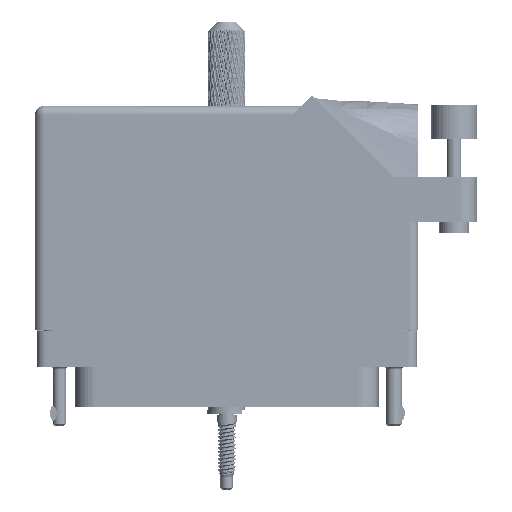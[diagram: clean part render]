
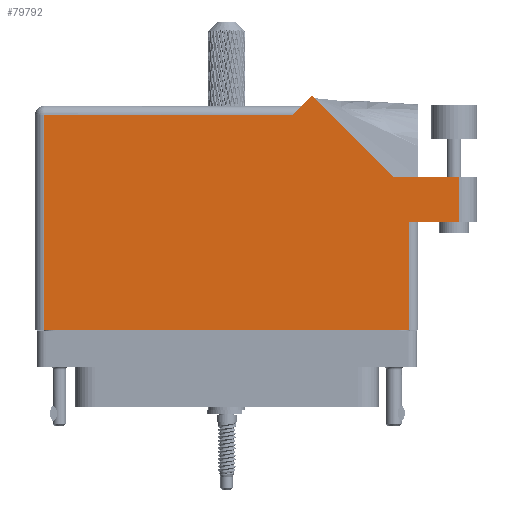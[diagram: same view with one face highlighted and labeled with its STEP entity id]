
A CAD part, front view. The second image highlights one B-rep face of the part: STEP entity #79792.
In plain terms, the highlighted face is planar.
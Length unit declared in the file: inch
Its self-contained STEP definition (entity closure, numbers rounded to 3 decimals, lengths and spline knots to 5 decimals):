
#1045 = CARTESIAN_POINT ( 'NONE',  ( -1.306, 1.43, 0.455 ) ) ;
#4242 = CARTESIAN_POINT ( 'NONE',  ( 1.581, 0.944, 0.455 ) ) ;
#14697 = ORIENTED_EDGE ( 'NONE', *, *, #37537, .T. ) ;
#15006 = DIRECTION ( 'NONE',  ( 1., 0., 0. ) ) ;
#15393 = CARTESIAN_POINT ( 'NONE',  ( 0.451, 1.368, 0.455 ) ) ;
#20619 = DIRECTION ( 'NONE',  ( 0., -1., 0. ) ) ;
#20991 = DIRECTION ( 'NONE',  ( -0.707, 0.707, 0. ) ) ;
#21075 = ORIENTED_EDGE ( 'NONE', *, *, #108436, .T. ) ;
#21555 = CARTESIAN_POINT ( 'NONE',  ( 1.244, 0.637, 0.455 ) ) ;
#22391 = VERTEX_POINT ( 'NONE', #112674 ) ;
#24322 = VECTOR ( 'NONE', #20619, 39.37008 ) ;
#25851 = VECTOR ( 'NONE', #105785, 39.37008 ) ;
#31049 = DIRECTION ( 'NONE',  ( 0., 0., -1. ) ) ;
#32817 = AXIS2_PLACEMENT_3D ( 'NONE', #1045, #31049, #50340 ) ;
#33758 = CARTESIAN_POINT ( 'NONE',  ( -1.244, -0.1, 0.455 ) ) ;
#33874 = CARTESIAN_POINT ( 'NONE',  ( 1.306, 0.637, 0.455 ) ) ;
#33957 = FACE_OUTER_BOUND ( 'NONE', #116750, .T. ) ;
#36675 = LINE ( 'NONE', #96003, #25851 ) ;
#37343 = VECTOR ( 'NONE', #15006, 39.37008 ) ;
#37527 = DIRECTION ( 'NONE',  ( -0.707, -0.707, 0. ) ) ;
#37537 = EDGE_CURVE ( 'NONE', #22391, #112021, #111509, .T. ) ;
#41765 = LINE ( 'NONE', #87621, #73941 ) ;
#42538 = ORIENTED_EDGE ( 'NONE', *, *, #68388, .T. ) ;
#42593 = VECTOR ( 'NONE', #88338, 39.37008 ) ;
#44472 = LINE ( 'NONE', #85574, #93372 ) ;
#46947 = LINE ( 'NONE', #94909, #120413 ) ;
#48667 = LINE ( 'NONE', #102746, #112873 ) ;
#48889 = VERTEX_POINT ( 'NONE', #4242 ) ;
#49794 = ORIENTED_EDGE ( 'NONE', *, *, #124087, .T. ) ;
#50340 = DIRECTION ( 'NONE',  ( -1., 0., 0. ) ) ;
#50769 = PLANE ( 'NONE',  #32817 ) ;
#54057 = VERTEX_POINT ( 'NONE', #117389 ) ;
#55526 = VERTEX_POINT ( 'NONE', #21555 ) ;
#56971 = CARTESIAN_POINT ( 'NONE',  ( 1.244, -0.1, 0.455 ) ) ;
#60945 = CARTESIAN_POINT ( 'NONE',  ( -1.244, -0.1, 0.455 ) ) ;
#61308 = VERTEX_POINT ( 'NONE', #111977 ) ;
#63271 = VERTEX_POINT ( 'NONE', #15393 ) ;
#68388 = EDGE_CURVE ( 'NONE', #63271, #22391, #36675, .T. ) ;
#72143 = ORIENTED_EDGE ( 'NONE', *, *, #79093, .T. ) ;
#73941 = VECTOR ( 'NONE', #37527, 39.37008 ) ;
#79093 = EDGE_CURVE ( 'NONE', #61308, #63271, #41765, .T. ) ;
#79255 = ORIENTED_EDGE ( 'NONE', *, *, #93267, .T. ) ;
#79792 = ADVANCED_FACE ( 'NONE', ( #33957 ), #50769, .F. ) ;
#79804 = ORIENTED_EDGE ( 'NONE', *, *, #101868, .T. ) ;
#81124 = EDGE_CURVE ( 'NONE', #48889, #54057, #44472, .T. ) ;
#85574 = CARTESIAN_POINT ( 'NONE',  ( 1.706, 0.944, 0.455 ) ) ;
#87621 = CARTESIAN_POINT ( 'NONE',  ( 0.513, 1.43, 0.455 ) ) ;
#88338 = DIRECTION ( 'NONE',  ( 0., 1., 0. ) ) ;
#89621 = VECTOR ( 'NONE', #20991, 39.37008 ) ;
#92226 = ORIENTED_EDGE ( 'NONE', *, *, #105990, .T. ) ;
#93267 = EDGE_CURVE ( 'NONE', #55526, #117722, #103076, .T. ) ;
#93372 = VECTOR ( 'NONE', #95356, 39.37008 ) ;
#93478 = VERTEX_POINT ( 'NONE', #56971 ) ;
#93817 = DIRECTION ( 'NONE',  ( 1., 0., 0. ) ) ;
#94564 = LINE ( 'NONE', #109145, #42593 ) ;
#94909 = CARTESIAN_POINT ( 'NONE',  ( 1.581, 0.944, 0.455 ) ) ;
#95356 = DIRECTION ( 'NONE',  ( -1., 0., 0. ) ) ;
#96003 = CARTESIAN_POINT ( 'NONE',  ( -1.306, 1.368, 0.455 ) ) ;
#98760 = LINE ( 'NONE', #118916, #89621 ) ;
#101868 = EDGE_CURVE ( 'NONE', #112021, #93478, #48667, .T. ) ;
#102746 = CARTESIAN_POINT ( 'NONE',  ( -1.306, -0.1, 0.455 ) ) ;
#103076 = LINE ( 'NONE', #33874, #37343 ) ;
#105785 = DIRECTION ( 'NONE',  ( -1., 0., 0. ) ) ;
#105990 = EDGE_CURVE ( 'NONE', #93478, #55526, #94564, .T. ) ;
#108436 = EDGE_CURVE ( 'NONE', #54057, #61308, #98760, .T. ) ;
#109145 = CARTESIAN_POINT ( 'NONE',  ( 1.244, 0.637, 0.455 ) ) ;
#111509 = LINE ( 'NONE', #60945, #24322 ) ;
#111977 = CARTESIAN_POINT ( 'NONE',  ( 0.58371, 1.50071, 0.455 ) ) ;
#112021 = VERTEX_POINT ( 'NONE', #33758 ) ;
#112674 = CARTESIAN_POINT ( 'NONE',  ( -1.244, 1.368, 0.455 ) ) ;
#112873 = VECTOR ( 'NONE', #93817, 39.37008 ) ;
#113150 = ORIENTED_EDGE ( 'NONE', *, *, #81124, .T. ) ;
#116305 = CARTESIAN_POINT ( 'NONE',  ( 1.581, 0.637, 0.455 ) ) ;
#116750 = EDGE_LOOP ( 'NONE', ( #79255, #49794, #113150, #21075, #72143, #42538, #14697, #79804, #92226 ) ) ;
#117389 = CARTESIAN_POINT ( 'NONE',  ( 1.14042, 0.944, 0.455 ) ) ;
#117722 = VERTEX_POINT ( 'NONE', #116305 ) ;
#118916 = CARTESIAN_POINT ( 'NONE',  ( 1.14042, 0.944, 0.455 ) ) ;
#120413 = VECTOR ( 'NONE', #125214, 39.37008 ) ;
#124087 = EDGE_CURVE ( 'NONE', #117722, #48889, #46947, .T. ) ;
#125214 = DIRECTION ( 'NONE',  ( 0., 1., 0. ) ) ;
